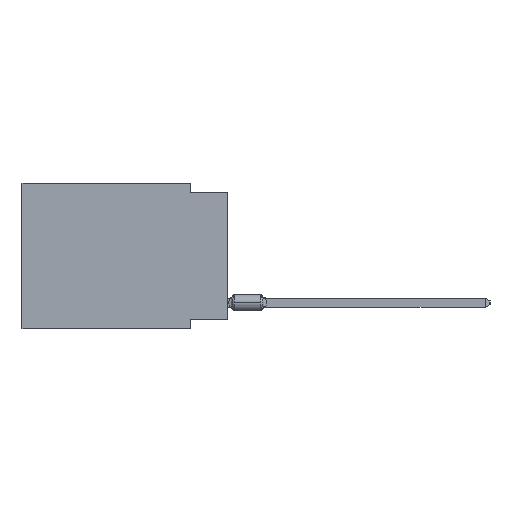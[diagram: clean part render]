
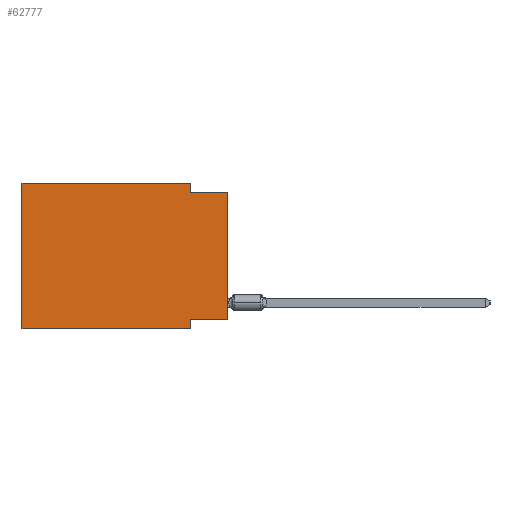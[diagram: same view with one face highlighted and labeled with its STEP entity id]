
A CAD part, left-side view. The second image highlights one B-rep face of the part: STEP entity #62777.
In plain terms, the highlighted planar face has unit normal (-1, 0, 0).
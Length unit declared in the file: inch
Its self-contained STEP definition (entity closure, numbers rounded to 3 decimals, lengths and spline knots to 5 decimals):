
#1810 = EDGE_CURVE ( 'NONE', #62840, #38594, #69086, .T. ) ;
#2614 = CARTESIAN_POINT ( 'NONE',  ( 0., 0., -0.025 ) ) ;
#3859 = LINE ( 'NONE', #40429, #54153 ) ;
#5634 = DIRECTION ( 'NONE',  ( 0., 0., -1. ) ) ;
#7238 = FACE_OUTER_BOUND ( 'NONE', #43353, .T. ) ;
#8852 = CARTESIAN_POINT ( 'NONE',  ( 0., 0.55, -0.39 ) ) ;
#13658 = VECTOR ( 'NONE', #25861, 39.37008 ) ;
#13926 = LINE ( 'NONE', #63261, #66746 ) ;
#14214 = CARTESIAN_POINT ( 'NONE',  ( 0., 0.55, 0. ) ) ;
#15892 = ORIENTED_EDGE ( 'NONE', *, *, #25848, .F. ) ;
#19565 = ORIENTED_EDGE ( 'NONE', *, *, #1810, .T. ) ;
#19970 = DIRECTION ( 'NONE',  ( 0., 0., -1. ) ) ;
#20342 = VERTEX_POINT ( 'NONE', #52428 ) ;
#20812 = DIRECTION ( 'NONE',  ( 0., 1., 0. ) ) ;
#20820 = CARTESIAN_POINT ( 'NONE',  ( 0., 0.55, 0. ) ) ;
#21187 = VECTOR ( 'NONE', #20812, 39.37008 ) ;
#21261 = CARTESIAN_POINT ( 'NONE',  ( 0., 0.55, 0. ) ) ;
#25848 = EDGE_CURVE ( 'NONE', #67169, #61505, #45486, .T. ) ;
#25861 = DIRECTION ( 'NONE',  ( 0., 0., -1. ) ) ;
#26381 = ORIENTED_EDGE ( 'NONE', *, *, #80561, .F. ) ;
#29914 = ORIENTED_EDGE ( 'NONE', *, *, #35407, .F. ) ;
#31318 = EDGE_CURVE ( 'NONE', #75976, #36247, #3859, .T. ) ;
#31591 = ORIENTED_EDGE ( 'NONE', *, *, #47533, .F. ) ;
#32018 = DIRECTION ( 'NONE',  ( 0., 0., 1. ) ) ;
#34670 = CARTESIAN_POINT ( 'NONE',  ( 0., 0.1, -0.025 ) ) ;
#35407 = EDGE_CURVE ( 'NONE', #61505, #75976, #45171, .T. ) ;
#36247 = VERTEX_POINT ( 'NONE', #2614 ) ;
#36455 = CARTESIAN_POINT ( 'NONE',  ( 0., 0.1, -0.39 ) ) ;
#38594 = VERTEX_POINT ( 'NONE', #63754 ) ;
#39304 = EDGE_CURVE ( 'NONE', #20342, #38594, #42255, .T. ) ;
#40179 = CARTESIAN_POINT ( 'NONE',  ( 0., 0., -0.365 ) ) ;
#40429 = CARTESIAN_POINT ( 'NONE',  ( 0., 0., -0.025 ) ) ;
#42255 = LINE ( 'NONE', #36455, #56895 ) ;
#43353 = EDGE_LOOP ( 'NONE', ( #67968, #60010, #29914, #15892, #31591, #19565, #81220, #26381 ) ) ;
#45171 = LINE ( 'NONE', #76416, #13658 ) ;
#45486 = LINE ( 'NONE', #20820, #47120 ) ;
#45902 = VERTEX_POINT ( 'NONE', #40179 ) ;
#47120 = VECTOR ( 'NONE', #70560, 39.37008 ) ;
#47533 = EDGE_CURVE ( 'NONE', #62840, #67169, #13926, .T. ) ;
#48606 = AXIS2_PLACEMENT_3D ( 'NONE', #14214, #64348, #19970 ) ;
#49575 = CARTESIAN_POINT ( 'NONE',  ( 0., 0.1, 0. ) ) ;
#49782 = DIRECTION ( 'NONE',  ( 0., -1., 0. ) ) ;
#51213 = VECTOR ( 'NONE', #49782, 39.37008 ) ;
#52428 = CARTESIAN_POINT ( 'NONE',  ( 0., 0.1, -0.365 ) ) ;
#54153 = VECTOR ( 'NONE', #78651, 39.37008 ) ;
#56895 = VECTOR ( 'NONE', #5634, 39.37008 ) ;
#57373 = PLANE ( 'NONE',  #48606 ) ;
#59428 = CARTESIAN_POINT ( 'NONE',  ( 0., 0., -0.365 ) ) ;
#60010 = ORIENTED_EDGE ( 'NONE', *, *, #31318, .F. ) ;
#60989 = CARTESIAN_POINT ( 'NONE',  ( 0., 0., 0. ) ) ;
#61388 = LINE ( 'NONE', #60989, #65194 ) ;
#61505 = VERTEX_POINT ( 'NONE', #49575 ) ;
#62777 = ADVANCED_FACE ( 'NONE', ( #7238 ), #57373, .F. ) ;
#62840 = VERTEX_POINT ( 'NONE', #8852 ) ;
#63261 = CARTESIAN_POINT ( 'NONE',  ( 0., 0.55, 0. ) ) ;
#63754 = CARTESIAN_POINT ( 'NONE',  ( 0., 0.1, -0.39 ) ) ;
#64348 = DIRECTION ( 'NONE',  ( 1., 0., 0. ) ) ;
#65194 = VECTOR ( 'NONE', #73721, 39.37008 ) ;
#66746 = VECTOR ( 'NONE', #32018, 39.37008 ) ;
#67169 = VERTEX_POINT ( 'NONE', #21261 ) ;
#67968 = ORIENTED_EDGE ( 'NONE', *, *, #69189, .T. ) ;
#68275 = CARTESIAN_POINT ( 'NONE',  ( 0., 0.55, -0.39 ) ) ;
#69086 = LINE ( 'NONE', #68275, #51213 ) ;
#69189 = EDGE_CURVE ( 'NONE', #45902, #36247, #61388, .T. ) ;
#70560 = DIRECTION ( 'NONE',  ( 0., -1., 0. ) ) ;
#73721 = DIRECTION ( 'NONE',  ( 0., 0., 1. ) ) ;
#75976 = VERTEX_POINT ( 'NONE', #34670 ) ;
#76416 = CARTESIAN_POINT ( 'NONE',  ( 0., 0.1, 0. ) ) ;
#78327 = LINE ( 'NONE', #59428, #21187 ) ;
#78651 = DIRECTION ( 'NONE',  ( 0., -1., 0. ) ) ;
#80561 = EDGE_CURVE ( 'NONE', #45902, #20342, #78327, .T. ) ;
#81220 = ORIENTED_EDGE ( 'NONE', *, *, #39304, .F. ) ;
